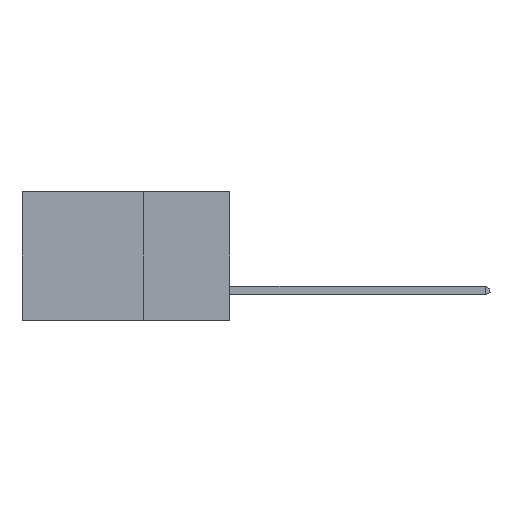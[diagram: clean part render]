
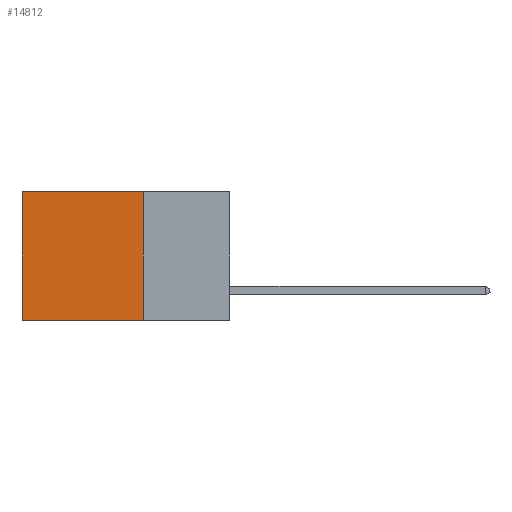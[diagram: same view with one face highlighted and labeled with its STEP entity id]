
A CAD part, left-side view. The second image highlights one B-rep face of the part: STEP entity #14812.
In plain terms, the highlighted planar face has unit normal (-1, 0, 0).
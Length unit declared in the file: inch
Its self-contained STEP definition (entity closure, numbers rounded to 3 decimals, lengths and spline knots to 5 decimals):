
#191 = EDGE_CURVE ( 'NONE', #6548, #15155, #12716, .T. ) ;
#603 = DIRECTION ( 'NONE',  ( 1., 0., 0. ) ) ;
#625 = CARTESIAN_POINT ( 'NONE',  ( 0.298, 0.25, -0.37 ) ) ;
#1592 = VECTOR ( 'NONE', #12040, 39.37008 ) ;
#1648 = EDGE_CURVE ( 'NONE', #8100, #15155, #13710, .T. ) ;
#2026 = CARTESIAN_POINT ( 'NONE',  ( 0.298, 0.25, 0. ) ) ;
#2430 = CARTESIAN_POINT ( 'NONE',  ( 0.298, 0.25, 0. ) ) ;
#2913 = CARTESIAN_POINT ( 'NONE',  ( 0.298, 0.6, 0. ) ) ;
#3263 = DIRECTION ( 'NONE',  ( 0., 1., 0. ) ) ;
#3448 = CARTESIAN_POINT ( 'NONE',  ( 0.298, 0.25, 0. ) ) ;
#4057 = CARTESIAN_POINT ( 'NONE',  ( 0.298, 0.6, -0.37 ) ) ;
#4320 = DIRECTION ( 'NONE',  ( 0., 0., -1. ) ) ;
#4491 = EDGE_LOOP ( 'NONE', ( #5718, #4546, #17487, #9546 ) ) ;
#4546 = ORIENTED_EDGE ( 'NONE', *, *, #1648, .F. ) ;
#4820 = LINE ( 'NONE', #11839, #9909 ) ;
#5718 = ORIENTED_EDGE ( 'NONE', *, *, #191, .T. ) ;
#6548 = VERTEX_POINT ( 'NONE', #16010 ) ;
#8100 = VERTEX_POINT ( 'NONE', #625 ) ;
#8916 = VECTOR ( 'NONE', #3263, 39.37008 ) ;
#9482 = EDGE_CURVE ( 'NONE', #9971, #6548, #12861, .T. ) ;
#9546 = ORIENTED_EDGE ( 'NONE', *, *, #9482, .T. ) ;
#9909 = VECTOR ( 'NONE', #12027, 39.37008 ) ;
#9971 = VERTEX_POINT ( 'NONE', #2430 ) ;
#10482 = DIRECTION ( 'NONE',  ( 0., 0., -1. ) ) ;
#11839 = CARTESIAN_POINT ( 'NONE',  ( 0.298, 0.25, 0. ) ) ;
#12027 = DIRECTION ( 'NONE',  ( 0., 0., -1. ) ) ;
#12040 = DIRECTION ( 'NONE',  ( 0., 1., 0. ) ) ;
#12716 = LINE ( 'NONE', #2913, #13351 ) ;
#12742 = AXIS2_PLACEMENT_3D ( 'NONE', #3448, #603, #10482 ) ;
#12861 = LINE ( 'NONE', #2026, #1592 ) ;
#13064 = PLANE ( 'NONE',  #12742 ) ;
#13276 = CARTESIAN_POINT ( 'NONE',  ( 0.298, 0.25, -0.37 ) ) ;
#13351 = VECTOR ( 'NONE', #4320, 39.37008 ) ;
#13710 = LINE ( 'NONE', #13276, #8916 ) ;
#14485 = EDGE_CURVE ( 'NONE', #9971, #8100, #4820, .T. ) ;
#14812 = ADVANCED_FACE ( 'NONE', ( #14899 ), #13064, .F. ) ;
#14899 = FACE_OUTER_BOUND ( 'NONE', #4491, .T. ) ;
#15155 = VERTEX_POINT ( 'NONE', #4057 ) ;
#16010 = CARTESIAN_POINT ( 'NONE',  ( 0.298, 0.6, 0. ) ) ;
#17487 = ORIENTED_EDGE ( 'NONE', *, *, #14485, .F. ) ;
